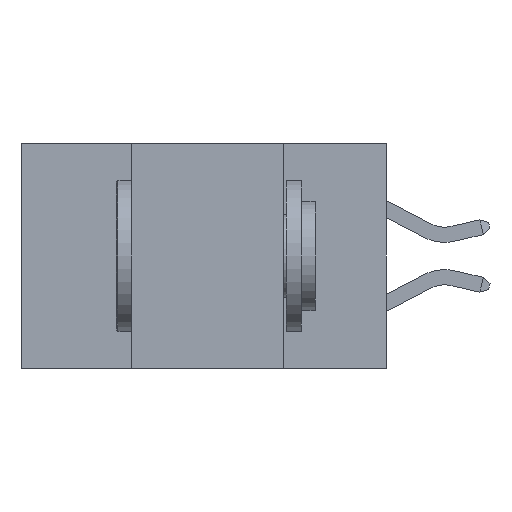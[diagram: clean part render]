
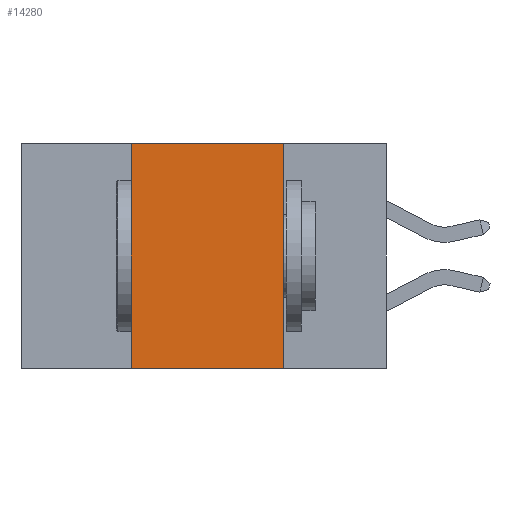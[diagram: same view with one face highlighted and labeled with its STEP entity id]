
A CAD part, left-side view. The second image highlights one B-rep face of the part: STEP entity #14280.
In plain terms, the highlighted planar face has unit normal (-1, 0, 0).
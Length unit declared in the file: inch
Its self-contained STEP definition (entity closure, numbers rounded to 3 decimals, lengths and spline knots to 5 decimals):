
#437 = DIRECTION ( 'NONE',  ( 1., 0., 0. ) ) ;
#1311 = LINE ( 'NONE', #14942, #13934 ) ;
#1682 = CARTESIAN_POINT ( 'NONE',  ( 0., 0.6, 0. ) ) ;
#1710 = LINE ( 'NONE', #8880, #11399 ) ;
#2557 = EDGE_CURVE ( 'NONE', #6724, #4807, #1710, .T. ) ;
#2602 = FACE_OUTER_BOUND ( 'NONE', #5479, .T. ) ;
#2847 = EDGE_CURVE ( 'NONE', #6724, #4363, #1311, .T. ) ;
#3831 = LINE ( 'NONE', #3937, #13102 ) ;
#3893 = DIRECTION ( 'NONE',  ( 0., -1., 0. ) ) ;
#3937 = CARTESIAN_POINT ( 'NONE',  ( 0., 0.6, 0. ) ) ;
#4096 = ORIENTED_EDGE ( 'NONE', *, *, #12005, .F. ) ;
#4363 = VERTEX_POINT ( 'NONE', #10973 ) ;
#4565 = VERTEX_POINT ( 'NONE', #9705 ) ;
#4735 = DIRECTION ( 'NONE',  ( 0., 0., -1. ) ) ;
#4807 = VERTEX_POINT ( 'NONE', #7674 ) ;
#4829 = CARTESIAN_POINT ( 'NONE',  ( 0., 0.17, -0.37 ) ) ;
#5479 = EDGE_LOOP ( 'NONE', ( #11239, #4096, #7094, #12956 ) ) ;
#6724 = VERTEX_POINT ( 'NONE', #9505 ) ;
#7094 = ORIENTED_EDGE ( 'NONE', *, *, #2847, .F. ) ;
#7491 = AXIS2_PLACEMENT_3D ( 'NONE', #1682, #437, #9367 ) ;
#7674 = CARTESIAN_POINT ( 'NONE',  ( 0., 0.17, -0.37 ) ) ;
#8462 = VECTOR ( 'NONE', #4735, 39.37008 ) ;
#8822 = DIRECTION ( 'NONE',  ( 0., -1., 0. ) ) ;
#8857 = LINE ( 'NONE', #4829, #8462 ) ;
#8880 = CARTESIAN_POINT ( 'NONE',  ( 0., 0.6, -0.37 ) ) ;
#9367 = DIRECTION ( 'NONE',  ( 0., 0., -1. ) ) ;
#9505 = CARTESIAN_POINT ( 'NONE',  ( 0., 0.42, -0.37 ) ) ;
#9705 = CARTESIAN_POINT ( 'NONE',  ( 0., 0.17, 0. ) ) ;
#10973 = CARTESIAN_POINT ( 'NONE',  ( 0., 0.42, 0. ) ) ;
#11239 = ORIENTED_EDGE ( 'NONE', *, *, #11862, .F. ) ;
#11399 = VECTOR ( 'NONE', #8822, 39.37008 ) ;
#11862 = EDGE_CURVE ( 'NONE', #4565, #4807, #8857, .T. ) ;
#12005 = EDGE_CURVE ( 'NONE', #4363, #4565, #3831, .T. ) ;
#12956 = ORIENTED_EDGE ( 'NONE', *, *, #2557, .T. ) ;
#13102 = VECTOR ( 'NONE', #3893, 39.37008 ) ;
#13934 = VECTOR ( 'NONE', #14702, 39.37008 ) ;
#14257 = PLANE ( 'NONE',  #7491 ) ;
#14280 = ADVANCED_FACE ( 'NONE', ( #2602 ), #14257, .F. ) ;
#14702 = DIRECTION ( 'NONE',  ( 0., 0., 1. ) ) ;
#14942 = CARTESIAN_POINT ( 'NONE',  ( 0., 0.42, -0.37 ) ) ;
